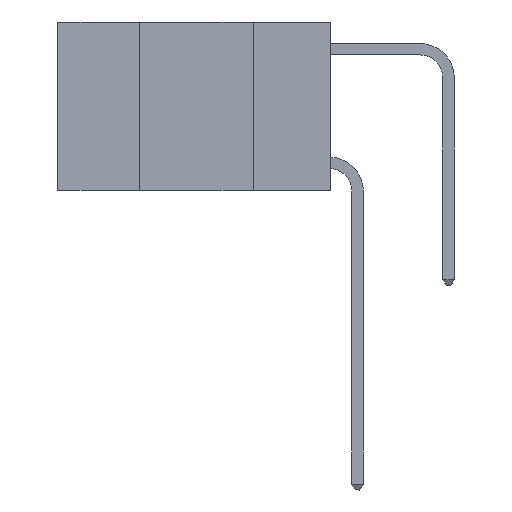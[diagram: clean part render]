
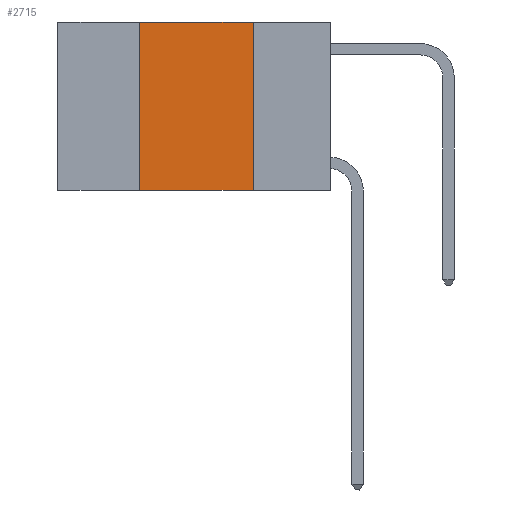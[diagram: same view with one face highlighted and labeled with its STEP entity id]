
A CAD part, left-side view. The second image highlights one B-rep face of the part: STEP entity #2715.
In plain terms, the highlighted planar face has unit normal (-1, 0, 0).
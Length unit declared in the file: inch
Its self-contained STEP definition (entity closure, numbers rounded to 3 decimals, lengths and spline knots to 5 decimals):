
#440 = FACE_OUTER_BOUND ( 'NONE', #4838, .T. ) ;
#723 = LINE ( 'NONE', #11935, #15919 ) ;
#748 = CARTESIAN_POINT ( 'NONE',  ( 0., 0.6, 0. ) ) ;
#1876 = DIRECTION ( 'NONE',  ( 0., -1., 0. ) ) ;
#2557 = LINE ( 'NONE', #12273, #5553 ) ;
#2715 = ADVANCED_FACE ( 'NONE', ( #440 ), #12240, .F. ) ;
#2816 = EDGE_CURVE ( 'NONE', #14690, #8038, #7076, .T. ) ;
#2939 = EDGE_CURVE ( 'NONE', #8038, #16821, #8205, .T. ) ;
#2969 = ORIENTED_EDGE ( 'NONE', *, *, #16928, .T. ) ;
#3691 = DIRECTION ( 'NONE',  ( 0., 0., -1. ) ) ;
#3913 = CARTESIAN_POINT ( 'NONE',  ( 0., 0.42, 0. ) ) ;
#4375 = CARTESIAN_POINT ( 'NONE',  ( 0., 0.17, -0.37 ) ) ;
#4588 = CARTESIAN_POINT ( 'NONE',  ( 0., 0.17, 0. ) ) ;
#4750 = ORIENTED_EDGE ( 'NONE', *, *, #2816, .F. ) ;
#4812 = VECTOR ( 'NONE', #15792, 39.37008 ) ;
#4838 = EDGE_LOOP ( 'NONE', ( #7406, #5082, #4750, #2969 ) ) ;
#5082 = ORIENTED_EDGE ( 'NONE', *, *, #2939, .F. ) ;
#5111 = AXIS2_PLACEMENT_3D ( 'NONE', #748, #13641, #5168 ) ;
#5168 = DIRECTION ( 'NONE',  ( 0., 0., -1. ) ) ;
#5424 = DIRECTION ( 'NONE',  ( 0., 0., 1. ) ) ;
#5553 = VECTOR ( 'NONE', #3691, 39.37008 ) ;
#6643 = VECTOR ( 'NONE', #5424, 39.37008 ) ;
#7076 = LINE ( 'NONE', #3913, #6643 ) ;
#7193 = CARTESIAN_POINT ( 'NONE',  ( 0., 0.42, -0.37 ) ) ;
#7356 = CARTESIAN_POINT ( 'NONE',  ( 0., 0.6, 0. ) ) ;
#7406 = ORIENTED_EDGE ( 'NONE', *, *, #10451, .F. ) ;
#8038 = VERTEX_POINT ( 'NONE', #10933 ) ;
#8205 = LINE ( 'NONE', #7356, #4812 ) ;
#10451 = EDGE_CURVE ( 'NONE', #16821, #15432, #2557, .T. ) ;
#10933 = CARTESIAN_POINT ( 'NONE',  ( 0., 0.42, 0. ) ) ;
#11935 = CARTESIAN_POINT ( 'NONE',  ( 0., 0.6, -0.37 ) ) ;
#12240 = PLANE ( 'NONE',  #5111 ) ;
#12273 = CARTESIAN_POINT ( 'NONE',  ( 0., 0.17, 0. ) ) ;
#13641 = DIRECTION ( 'NONE',  ( 1., 0., 0. ) ) ;
#14690 = VERTEX_POINT ( 'NONE', #7193 ) ;
#15432 = VERTEX_POINT ( 'NONE', #4375 ) ;
#15792 = DIRECTION ( 'NONE',  ( 0., -1., 0. ) ) ;
#15919 = VECTOR ( 'NONE', #1876, 39.37008 ) ;
#16821 = VERTEX_POINT ( 'NONE', #4588 ) ;
#16928 = EDGE_CURVE ( 'NONE', #14690, #15432, #723, .T. ) ;
